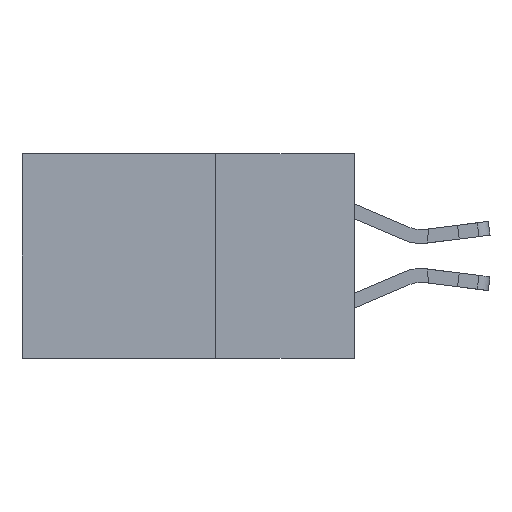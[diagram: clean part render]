
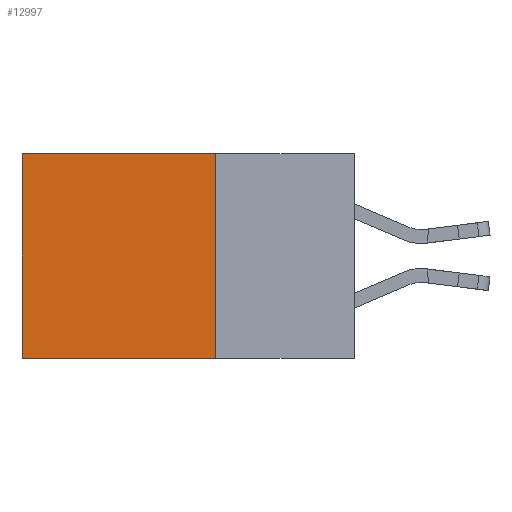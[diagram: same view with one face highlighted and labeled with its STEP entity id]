
A CAD part, left-side view. The second image highlights one B-rep face of the part: STEP entity #12997.
In plain terms, the highlighted planar face has unit normal (-1, 0, 0).
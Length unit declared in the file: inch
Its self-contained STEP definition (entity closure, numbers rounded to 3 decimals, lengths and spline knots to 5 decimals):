
#200 = ORIENTED_EDGE ( 'NONE', *, *, #10869, .T. ) ;
#1616 = PLANE ( 'NONE',  #16669 ) ;
#1629 = LINE ( 'NONE', #5359, #8095 ) ;
#2955 = DIRECTION ( 'NONE',  ( 0., 0., -1. ) ) ;
#3247 = DIRECTION ( 'NONE',  ( 0., 0., -1. ) ) ;
#3344 = EDGE_CURVE ( 'NONE', #11635, #9911, #14065, .T. ) ;
#3389 = LINE ( 'NONE', #14252, #13665 ) ;
#3612 = VERTEX_POINT ( 'NONE', #5001 ) ;
#3630 = EDGE_LOOP ( 'NONE', ( #4253, #16049, #10857, #200 ) ) ;
#3886 = LINE ( 'NONE', #5230, #13762 ) ;
#4253 = ORIENTED_EDGE ( 'NONE', *, *, #3344, .T. ) ;
#5001 = CARTESIAN_POINT ( 'NONE',  ( 0.298, 0.25, -0.37 ) ) ;
#5228 = DIRECTION ( 'NONE',  ( 0., 0., -1. ) ) ;
#5230 = CARTESIAN_POINT ( 'NONE',  ( 0.298, 0.25, -0.37 ) ) ;
#5359 = CARTESIAN_POINT ( 'NONE',  ( 0.298, 0.25, 0. ) ) ;
#5824 = FACE_OUTER_BOUND ( 'NONE', #3630, .T. ) ;
#7185 = VECTOR ( 'NONE', #3247, 39.37008 ) ;
#7904 = CARTESIAN_POINT ( 'NONE',  ( 0.298, 0.25, 0. ) ) ;
#8095 = VECTOR ( 'NONE', #14370, 39.37008 ) ;
#8217 = CARTESIAN_POINT ( 'NONE',  ( 0.298, 0.6, 0. ) ) ;
#9532 = VERTEX_POINT ( 'NONE', #7904 ) ;
#9633 = CARTESIAN_POINT ( 'NONE',  ( 0.298, 0.6, 0. ) ) ;
#9911 = VERTEX_POINT ( 'NONE', #12486 ) ;
#10678 = DIRECTION ( 'NONE',  ( 1., 0., 0. ) ) ;
#10857 = ORIENTED_EDGE ( 'NONE', *, *, #14708, .F. ) ;
#10869 = EDGE_CURVE ( 'NONE', #9532, #11635, #1629, .T. ) ;
#11409 = EDGE_CURVE ( 'NONE', #3612, #9911, #3886, .T. ) ;
#11635 = VERTEX_POINT ( 'NONE', #8217 ) ;
#11955 = CARTESIAN_POINT ( 'NONE',  ( 0.298, 0.25, 0. ) ) ;
#12486 = CARTESIAN_POINT ( 'NONE',  ( 0.298, 0.6, -0.37 ) ) ;
#12997 = ADVANCED_FACE ( 'NONE', ( #5824 ), #1616, .F. ) ;
#13665 = VECTOR ( 'NONE', #5228, 39.37008 ) ;
#13762 = VECTOR ( 'NONE', #15555, 39.37008 ) ;
#14065 = LINE ( 'NONE', #9633, #7185 ) ;
#14252 = CARTESIAN_POINT ( 'NONE',  ( 0.298, 0.25, 0. ) ) ;
#14370 = DIRECTION ( 'NONE',  ( 0., 1., 0. ) ) ;
#14708 = EDGE_CURVE ( 'NONE', #9532, #3612, #3389, .T. ) ;
#15555 = DIRECTION ( 'NONE',  ( 0., 1., 0. ) ) ;
#16049 = ORIENTED_EDGE ( 'NONE', *, *, #11409, .F. ) ;
#16669 = AXIS2_PLACEMENT_3D ( 'NONE', #11955, #10678, #2955 ) ;
